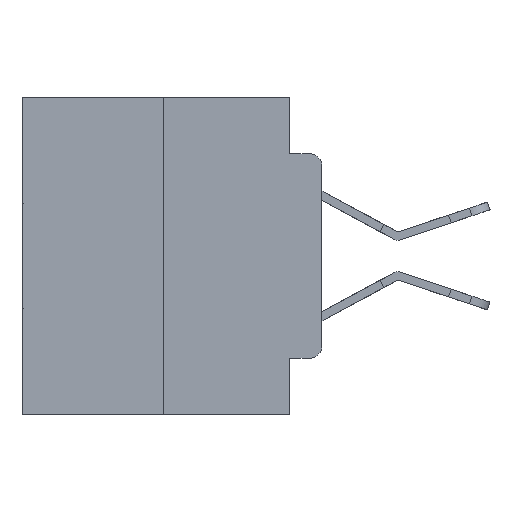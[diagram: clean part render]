
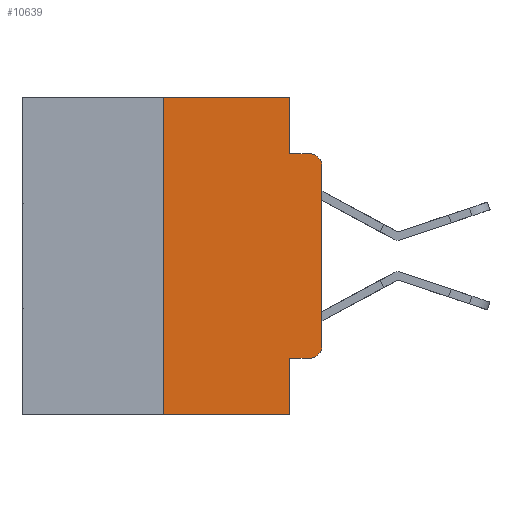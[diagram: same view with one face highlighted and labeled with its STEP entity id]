
A CAD part, left-side view. The second image highlights one B-rep face of the part: STEP entity #10639.
In plain terms, the highlighted planar face has unit normal (-1, 0, 0).
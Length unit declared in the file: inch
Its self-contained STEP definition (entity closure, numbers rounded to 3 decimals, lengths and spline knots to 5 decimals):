
#256 = DIRECTION ( 'NONE',  ( 0., 0., -1. ) ) ;
#356 = EDGE_CURVE ( 'NONE', #27050, #4112, #23427, .T. ) ;
#563 = CARTESIAN_POINT ( 'NONE',  ( 0., 0.02, -0.0885 ) ) ;
#1250 = VERTEX_POINT ( 'NONE', #19232 ) ;
#1392 = ORIENTED_EDGE ( 'NONE', *, *, #16206, .F. ) ;
#2058 = DIRECTION ( 'NONE',  ( 0., -1., 0. ) ) ;
#2657 = LINE ( 'NONE', #7601, #25461 ) ;
#2840 = ORIENTED_EDGE ( 'NONE', *, *, #21280, .T. ) ;
#3417 = VERTEX_POINT ( 'NONE', #22584 ) ;
#3992 = VERTEX_POINT ( 'NONE', #15452 ) ;
#4112 = VERTEX_POINT ( 'NONE', #15487 ) ;
#4381 = ORIENTED_EDGE ( 'NONE', *, *, #12585, .T. ) ;
#4763 = DIRECTION ( 'NONE',  ( 0., 0., 1. ) ) ;
#4789 = EDGE_CURVE ( 'NONE', #16197, #11272, #19116, .T. ) ;
#4905 = DIRECTION ( 'NONE',  ( 1., 0., 0. ) ) ;
#5105 = DIRECTION ( 'NONE',  ( 0., 0., 1. ) ) ;
#5454 = ORIENTED_EDGE ( 'NONE', *, *, #29162, .T. ) ;
#5819 = ORIENTED_EDGE ( 'NONE', *, *, #356, .F. ) ;
#7114 = CARTESIAN_POINT ( 'NONE',  ( 0., 0.25, 0. ) ) ;
#7601 = CARTESIAN_POINT ( 'NONE',  ( 0., 0., 0. ) ) ;
#7621 = AXIS2_PLACEMENT_3D ( 'NONE', #27579, #14258, #256 ) ;
#8417 = CARTESIAN_POINT ( 'NONE',  ( 0., 0.25, 0. ) ) ;
#8873 = ORIENTED_EDGE ( 'NONE', *, *, #4789, .F. ) ;
#8936 = ORIENTED_EDGE ( 'NONE', *, *, #10105, .F. ) ;
#9023 = VECTOR ( 'NONE', #9371, 39.37008 ) ;
#9371 = DIRECTION ( 'NONE',  ( 0., 0., -1. ) ) ;
#9548 = PLANE ( 'NONE',  #26001 ) ;
#9719 = ORIENTED_EDGE ( 'NONE', *, *, #23662, .F. ) ;
#10105 = EDGE_CURVE ( 'NONE', #15821, #3992, #20300, .T. ) ;
#10597 = ORIENTED_EDGE ( 'NONE', *, *, #22147, .T. ) ;
#10639 = ADVANCED_FACE ( 'NONE', ( #28980 ), #9548, .F. ) ;
#11272 = VERTEX_POINT ( 'NONE', #563 ) ;
#11738 = CARTESIAN_POINT ( 'NONE',  ( 0., 0.02, -0.1085 ) ) ;
#12240 = VECTOR ( 'NONE', #4763, 39.37008 ) ;
#12303 = CARTESIAN_POINT ( 'NONE',  ( 0., 0.051, -0.4115 ) ) ;
#12585 = EDGE_CURVE ( 'NONE', #1250, #21312, #2657, .T. ) ;
#12669 = CARTESIAN_POINT ( 'NONE',  ( 0., 0., -0.1085 ) ) ;
#13184 = VECTOR ( 'NONE', #14136, 39.37008 ) ;
#14063 = DIRECTION ( 'NONE',  ( 0., 0., -1. ) ) ;
#14136 = DIRECTION ( 'NONE',  ( 0., -1., 0. ) ) ;
#14258 = DIRECTION ( 'NONE',  ( -1., 0., 0. ) ) ;
#14785 = DIRECTION ( 'NONE',  ( 0., -1., 0. ) ) ;
#15452 = CARTESIAN_POINT ( 'NONE',  ( 0., 0.051, -0.5 ) ) ;
#15487 = CARTESIAN_POINT ( 'NONE',  ( 0., 0.051, 0. ) ) ;
#15821 = VERTEX_POINT ( 'NONE', #12303 ) ;
#16197 = VERTEX_POINT ( 'NONE', #20728 ) ;
#16206 = EDGE_CURVE ( 'NONE', #3417, #27050, #24170, .T. ) ;
#16304 = AXIS2_PLACEMENT_3D ( 'NONE', #11738, #27384, #14063 ) ;
#16860 = ORIENTED_EDGE ( 'NONE', *, *, #24220, .T. ) ;
#19116 = LINE ( 'NONE', #27464, #13184 ) ;
#19222 = CARTESIAN_POINT ( 'NONE',  ( 0., 0.473, -0.5 ) ) ;
#19232 = CARTESIAN_POINT ( 'NONE',  ( 0., 0., -0.3915 ) ) ;
#19411 = DIRECTION ( 'NONE',  ( 0., 0., -1. ) ) ;
#20076 = CIRCLE ( 'NONE', #16304, 0.02 ) ;
#20200 = CIRCLE ( 'NONE', #7621, 0.02 ) ;
#20300 = LINE ( 'NONE', #23826, #25565 ) ;
#20728 = CARTESIAN_POINT ( 'NONE',  ( 0., 0.051, -0.0885 ) ) ;
#20844 = LINE ( 'NONE', #19222, #26783 ) ;
#20875 = DIRECTION ( 'NONE',  ( 0., 0., -1. ) ) ;
#21280 = EDGE_CURVE ( 'NONE', #3417, #3992, #20844, .T. ) ;
#21312 = VERTEX_POINT ( 'NONE', #12669 ) ;
#21326 = VECTOR ( 'NONE', #2058, 39.37008 ) ;
#22147 = EDGE_CURVE ( 'NONE', #21312, #11272, #20076, .T. ) ;
#22584 = CARTESIAN_POINT ( 'NONE',  ( 0., 0.25, -0.5 ) ) ;
#22757 = CARTESIAN_POINT ( 'NONE',  ( 0., 0.051, 0. ) ) ;
#23427 = LINE ( 'NONE', #28410, #29259 ) ;
#23662 = EDGE_CURVE ( 'NONE', #4112, #16197, #26972, .T. ) ;
#23826 = CARTESIAN_POINT ( 'NONE',  ( 0., 0.051, 0. ) ) ;
#24170 = LINE ( 'NONE', #7114, #12240 ) ;
#24220 = EDGE_CURVE ( 'NONE', #15821, #29044, #27245, .T. ) ;
#25291 = CARTESIAN_POINT ( 'NONE',  ( 0., 0.473, 0. ) ) ;
#25461 = VECTOR ( 'NONE', #5105, 39.37008 ) ;
#25565 = VECTOR ( 'NONE', #19411, 39.37008 ) ;
#26001 = AXIS2_PLACEMENT_3D ( 'NONE', #25291, #4905, #20875 ) ;
#26783 = VECTOR ( 'NONE', #14785, 39.37008 ) ;
#26972 = LINE ( 'NONE', #22757, #9023 ) ;
#27050 = VERTEX_POINT ( 'NONE', #8417 ) ;
#27245 = LINE ( 'NONE', #29173, #21326 ) ;
#27384 = DIRECTION ( 'NONE',  ( -1., 0., 0. ) ) ;
#27464 = CARTESIAN_POINT ( 'NONE',  ( 0., 0.051, -0.0885 ) ) ;
#27579 = CARTESIAN_POINT ( 'NONE',  ( 0., 0.02, -0.3915 ) ) ;
#27875 = EDGE_LOOP ( 'NONE', ( #4381, #10597, #8873, #9719, #5819, #1392, #2840, #8936, #16860, #5454 ) ) ;
#28166 = DIRECTION ( 'NONE',  ( 0., -1., 0. ) ) ;
#28410 = CARTESIAN_POINT ( 'NONE',  ( 0., 0.473, 0. ) ) ;
#28980 = FACE_OUTER_BOUND ( 'NONE', #27875, .T. ) ;
#29044 = VERTEX_POINT ( 'NONE', #29172 ) ;
#29162 = EDGE_CURVE ( 'NONE', #29044, #1250, #20200, .T. ) ;
#29172 = CARTESIAN_POINT ( 'NONE',  ( 0., 0.02, -0.4115 ) ) ;
#29173 = CARTESIAN_POINT ( 'NONE',  ( 0., 0.051, -0.4115 ) ) ;
#29259 = VECTOR ( 'NONE', #28166, 39.37008 ) ;
